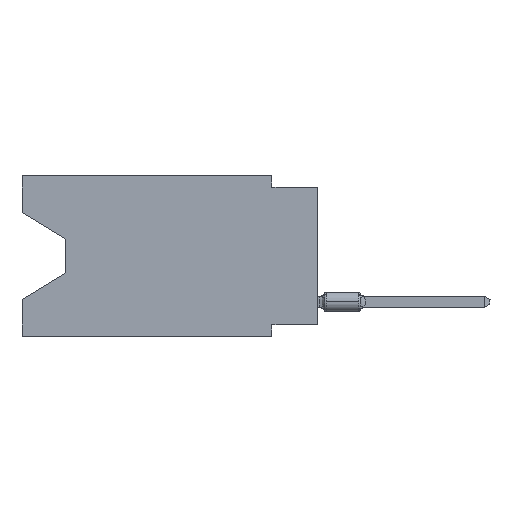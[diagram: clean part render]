
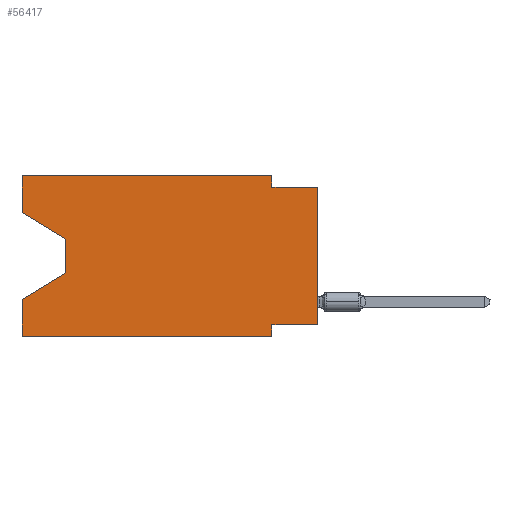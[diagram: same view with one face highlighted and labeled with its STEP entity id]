
A CAD part, left-side view. The second image highlights one B-rep face of the part: STEP entity #56417.
In plain terms, the highlighted planar face has unit normal (-1, 0, 0).
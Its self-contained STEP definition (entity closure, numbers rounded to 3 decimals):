
#841 = VERTEX_POINT ( 'NONE', #7107 ) ;
#898 = ORIENTED_EDGE ( 'NONE', *, *, #32333, .T. ) ;
#1056 = LINE ( 'NONE', #52514, #64758 ) ;
#1256 = LINE ( 'NONE', #38281, #68787 ) ;
#1265 = DIRECTION ( 'NONE',  ( 0., -1., 0. ) ) ;
#1745 = AXIS2_PLACEMENT_3D ( 'NONE', #27624, #56980, #20387 ) ;
#1980 = VECTOR ( 'NONE', #45403, 1000. ) ;
#2632 = DIRECTION ( 'NONE',  ( 0., 0., 1. ) ) ;
#2686 = CARTESIAN_POINT ( 'NONE',  ( 0., 16.383, -8.89 ) ) ;
#2883 = VERTEX_POINT ( 'NONE', #82171 ) ;
#3574 = VERTEX_POINT ( 'NONE', #66078 ) ;
#5426 = DIRECTION ( 'NONE',  ( 0., 0.855, -0.519 ) ) ;
#5758 = VERTEX_POINT ( 'NONE', #11453 ) ;
#6172 = EDGE_CURVE ( 'NONE', #2883, #16164, #63159, .T. ) ;
#7107 = CARTESIAN_POINT ( 'NONE',  ( 0., 2.54, -0.635 ) ) ;
#7755 = EDGE_CURVE ( 'NONE', #15573, #34165, #86931, .T. ) ;
#10300 = VECTOR ( 'NONE', #11881, 1000. ) ;
#11453 = CARTESIAN_POINT ( 'NONE',  ( 0., 2.54, 0. ) ) ;
#11881 = DIRECTION ( 'NONE',  ( 0., 0., 1. ) ) ;
#12474 = EDGE_CURVE ( 'NONE', #14062, #75719, #1056, .T. ) ;
#12733 = FACE_OUTER_BOUND ( 'NONE', #19906, .T. ) ;
#14062 = VERTEX_POINT ( 'NONE', #89990 ) ;
#15573 = VERTEX_POINT ( 'NONE', #91677 ) ;
#16164 = VERTEX_POINT ( 'NONE', #17261 ) ;
#17261 = CARTESIAN_POINT ( 'NONE',  ( 0., 16.383, -6.852 ) ) ;
#18121 = ORIENTED_EDGE ( 'NONE', *, *, #70461, .T. ) ;
#19906 = EDGE_LOOP ( 'NONE', ( #82660, #898, #61512, #87342, #72586, #70840, #78874, #18121, #46059, #61416, #90846, #95003 ) ) ;
#20387 = DIRECTION ( 'NONE',  ( 0., 0., -1. ) ) ;
#24020 = EDGE_CURVE ( 'NONE', #72420, #34165, #45990, .T. ) ;
#25357 = CARTESIAN_POINT ( 'NONE',  ( 0., 16.383, 0. ) ) ;
#27624 = CARTESIAN_POINT ( 'NONE',  ( 0., 16.383, 0. ) ) ;
#28710 = DIRECTION ( 'NONE',  ( 0., 0., -1. ) ) ;
#32324 = VECTOR ( 'NONE', #44210, 1000. ) ;
#32333 = EDGE_CURVE ( 'NONE', #75719, #2883, #1256, .T. ) ;
#34165 = VERTEX_POINT ( 'NONE', #73062 ) ;
#37935 = LINE ( 'NONE', #89401, #32324 ) ;
#38281 = CARTESIAN_POINT ( 'NONE',  ( 0., 13.97, -3.505 ) ) ;
#38698 = CARTESIAN_POINT ( 'NONE',  ( 0., 16.383, 0. ) ) ;
#39178 = VECTOR ( 'NONE', #57173, 1000. ) ;
#39532 = EDGE_CURVE ( 'NONE', #3574, #15573, #37935, .T. ) ;
#40418 = DIRECTION ( 'NONE',  ( 0., -1., 0. ) ) ;
#40588 = EDGE_CURVE ( 'NONE', #5758, #841, #59830, .T. ) ;
#44210 = DIRECTION ( 'NONE',  ( 0., 1., 0. ) ) ;
#44303 = DIRECTION ( 'NONE',  ( 0., -1., 0. ) ) ;
#45403 = DIRECTION ( 'NONE',  ( 0., 0., -1. ) ) ;
#45990 = LINE ( 'NONE', #59940, #70738 ) ;
#46059 = ORIENTED_EDGE ( 'NONE', *, *, #63809, .F. ) ;
#48120 = CARTESIAN_POINT ( 'NONE',  ( 0., 16.383, 0. ) ) ;
#50975 = EDGE_CURVE ( 'NONE', #80431, #5758, #77919, .T. ) ;
#51321 = CARTESIAN_POINT ( 'NONE',  ( 0., 2.54, -8.89 ) ) ;
#52514 = CARTESIAN_POINT ( 'NONE',  ( 0., 16.383, -2.038 ) ) ;
#52620 = CARTESIAN_POINT ( 'NONE',  ( 0., 2.54, 0. ) ) ;
#52719 = DIRECTION ( 'NONE',  ( 0., 0., -1. ) ) ;
#52937 = LINE ( 'NONE', #80859, #62735 ) ;
#56417 = ADVANCED_FACE ( 'NONE', ( #12733 ), #72364, .F. ) ;
#56980 = DIRECTION ( 'NONE',  ( 1., 0., 0. ) ) ;
#57173 = DIRECTION ( 'NONE',  ( 0., 0., 1. ) ) ;
#59248 = DIRECTION ( 'NONE',  ( 0., -0.855, -0.519 ) ) ;
#59830 = LINE ( 'NONE', #52620, #1980 ) ;
#59940 = CARTESIAN_POINT ( 'NONE',  ( 0., 16.383, -8.89 ) ) ;
#61416 = ORIENTED_EDGE ( 'NONE', *, *, #40588, .F. ) ;
#61512 = ORIENTED_EDGE ( 'NONE', *, *, #6172, .T. ) ;
#62735 = VECTOR ( 'NONE', #44303, 1000. ) ;
#63159 = LINE ( 'NONE', #77593, #67119 ) ;
#63809 = EDGE_CURVE ( 'NONE', #841, #79710, #52937, .T. ) ;
#64157 = VECTOR ( 'NONE', #40418, 1000. ) ;
#64758 = VECTOR ( 'NONE', #59248, 1000. ) ;
#66078 = CARTESIAN_POINT ( 'NONE',  ( 0., 0., -8.255 ) ) ;
#67119 = VECTOR ( 'NONE', #5426, 1000. ) ;
#67581 = LINE ( 'NONE', #38698, #67675 ) ;
#67675 = VECTOR ( 'NONE', #2632, 1000. ) ;
#68787 = VECTOR ( 'NONE', #52719, 1000. ) ;
#70461 = EDGE_CURVE ( 'NONE', #3574, #79710, #80726, .T. ) ;
#70738 = VECTOR ( 'NONE', #1265, 1000. ) ;
#70840 = ORIENTED_EDGE ( 'NONE', *, *, #7755, .F. ) ;
#71932 = EDGE_CURVE ( 'NONE', #14062, #80431, #91284, .T. ) ;
#72364 = PLANE ( 'NONE',  #1745 ) ;
#72420 = VERTEX_POINT ( 'NONE', #2686 ) ;
#72586 = ORIENTED_EDGE ( 'NONE', *, *, #24020, .T. ) ;
#73062 = CARTESIAN_POINT ( 'NONE',  ( 0., 2.54, -8.89 ) ) ;
#73143 = CARTESIAN_POINT ( 'NONE',  ( 0., 0., -0.635 ) ) ;
#73506 = CARTESIAN_POINT ( 'NONE',  ( 0., 0., 0. ) ) ;
#75719 = VERTEX_POINT ( 'NONE', #78725 ) ;
#77593 = CARTESIAN_POINT ( 'NONE',  ( 0., 13.97, -5.385 ) ) ;
#77919 = LINE ( 'NONE', #48120, #64157 ) ;
#78725 = CARTESIAN_POINT ( 'NONE',  ( 0., 13.97, -3.505 ) ) ;
#78874 = ORIENTED_EDGE ( 'NONE', *, *, #39532, .F. ) ;
#79085 = CARTESIAN_POINT ( 'NONE',  ( 0., 16.383, 0. ) ) ;
#79710 = VERTEX_POINT ( 'NONE', #73143 ) ;
#80431 = VERTEX_POINT ( 'NONE', #79085 ) ;
#80726 = LINE ( 'NONE', #73506, #39178 ) ;
#80859 = CARTESIAN_POINT ( 'NONE',  ( 0., 0., -0.635 ) ) ;
#82171 = CARTESIAN_POINT ( 'NONE',  ( 0., 13.97, -5.385 ) ) ;
#82660 = ORIENTED_EDGE ( 'NONE', *, *, #12474, .T. ) ;
#86931 = LINE ( 'NONE', #51321, #93400 ) ;
#87342 = ORIENTED_EDGE ( 'NONE', *, *, #88906, .F. ) ;
#88906 = EDGE_CURVE ( 'NONE', #72420, #16164, #67581, .T. ) ;
#89401 = CARTESIAN_POINT ( 'NONE',  ( 0., 0., -8.255 ) ) ;
#89990 = CARTESIAN_POINT ( 'NONE',  ( 0., 16.383, -2.038 ) ) ;
#90846 = ORIENTED_EDGE ( 'NONE', *, *, #50975, .F. ) ;
#91284 = LINE ( 'NONE', #25357, #10300 ) ;
#91677 = CARTESIAN_POINT ( 'NONE',  ( 0., 2.54, -8.255 ) ) ;
#93400 = VECTOR ( 'NONE', #28710, 1000. ) ;
#95003 = ORIENTED_EDGE ( 'NONE', *, *, #71932, .F. ) ;
